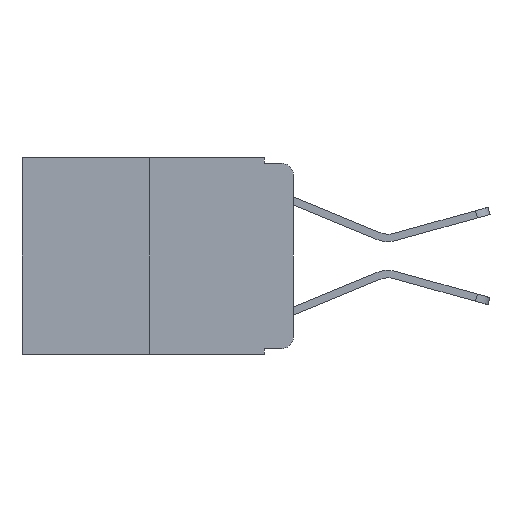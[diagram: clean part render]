
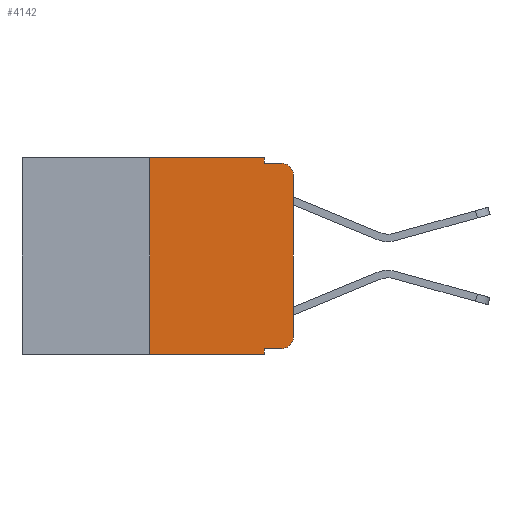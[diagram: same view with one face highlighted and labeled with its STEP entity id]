
A CAD part, left-side view. The second image highlights one B-rep face of the part: STEP entity #4142.
In plain terms, the highlighted planar face has unit normal (-1, 0, 0).
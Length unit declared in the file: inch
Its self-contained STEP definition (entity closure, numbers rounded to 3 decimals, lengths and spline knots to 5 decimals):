
#37 = DIRECTION ( 'NONE',  ( 0., -1., 0. ) ) ;
#138 = VECTOR ( 'NONE', #4565, 39.37008 ) ;
#332 = VERTEX_POINT ( 'NONE', #5326 ) ;
#410 = ORIENTED_EDGE ( 'NONE', *, *, #5003, .F. ) ;
#498 = VECTOR ( 'NONE', #1912, 39.37008 ) ;
#729 = EDGE_CURVE ( 'NONE', #332, #1767, #4614, .T. ) ;
#744 = LINE ( 'NONE', #3765, #852 ) ;
#795 = DIRECTION ( 'NONE',  ( 0., -1., 0. ) ) ;
#852 = VECTOR ( 'NONE', #9876, 39.37008 ) ;
#987 = EDGE_CURVE ( 'NONE', #9604, #3846, #1211, .T. ) ;
#1060 = CARTESIAN_POINT ( 'NONE',  ( 0., 0., 0. ) ) ;
#1211 = LINE ( 'NONE', #1060, #498 ) ;
#1225 = DIRECTION ( 'NONE',  ( 0., 0., -1. ) ) ;
#1314 = CARTESIAN_POINT ( 'NONE',  ( 0., 0.02, -0.03 ) ) ;
#1370 = PLANE ( 'NONE',  #2198 ) ;
#1767 = VERTEX_POINT ( 'NONE', #5515 ) ;
#1862 = ORIENTED_EDGE ( 'NONE', *, *, #2819, .F. ) ;
#1912 = DIRECTION ( 'NONE',  ( 0., 0., 1. ) ) ;
#2183 = EDGE_CURVE ( 'NONE', #1767, #5302, #744, .T. ) ;
#2198 = AXIS2_PLACEMENT_3D ( 'NONE', #9045, #6063, #7511 ) ;
#2219 = VECTOR ( 'NONE', #37, 39.37008 ) ;
#2294 = CARTESIAN_POINT ( 'NONE',  ( 0., 0.051, -0.01 ) ) ;
#2358 = LINE ( 'NONE', #4628, #5324 ) ;
#2541 = LINE ( 'NONE', #4808, #7480 ) ;
#2587 = DIRECTION ( 'NONE',  ( 0., 0., -1. ) ) ;
#2742 = ORIENTED_EDGE ( 'NONE', *, *, #3540, .T. ) ;
#2819 = EDGE_CURVE ( 'NONE', #7942, #332, #5285, .T. ) ;
#2828 = DIRECTION ( 'NONE',  ( 0., 0., 1. ) ) ;
#2835 = CIRCLE ( 'NONE', #9376, 0.02 ) ;
#2841 = DIRECTION ( 'NONE',  ( 0., 0., -1. ) ) ;
#3342 = EDGE_CURVE ( 'NONE', #9319, #7712, #2541, .T. ) ;
#3540 = EDGE_CURVE ( 'NONE', #7243, #9604, #2835, .T. ) ;
#3765 = CARTESIAN_POINT ( 'NONE',  ( 0., 0.051, 0. ) ) ;
#3846 = VERTEX_POINT ( 'NONE', #4092 ) ;
#3925 = CARTESIAN_POINT ( 'NONE',  ( 0., 0.051, -0.333 ) ) ;
#4092 = CARTESIAN_POINT ( 'NONE',  ( 0., 0., -0.03 ) ) ;
#4142 = ADVANCED_FACE ( 'NONE', ( #7606 ), #1370, .F. ) ;
#4565 = DIRECTION ( 'NONE',  ( 0., -1., 0. ) ) ;
#4577 = CARTESIAN_POINT ( 'NONE',  ( 0., 0., -0.313 ) ) ;
#4614 = LINE ( 'NONE', #5931, #7427 ) ;
#4628 = CARTESIAN_POINT ( 'NONE',  ( 0., 0.051, -0.333 ) ) ;
#4680 = ORIENTED_EDGE ( 'NONE', *, *, #2183, .F. ) ;
#4808 = CARTESIAN_POINT ( 'NONE',  ( 0., 0.051, 0. ) ) ;
#5003 = EDGE_CURVE ( 'NONE', #5302, #6569, #8308, .T. ) ;
#5243 = CARTESIAN_POINT ( 'NONE',  ( 0., 0.25, 0. ) ) ;
#5263 = EDGE_CURVE ( 'NONE', #3846, #6569, #6538, .T. ) ;
#5285 = LINE ( 'NONE', #5243, #8584 ) ;
#5302 = VERTEX_POINT ( 'NONE', #8946 ) ;
#5324 = VECTOR ( 'NONE', #795, 39.37008 ) ;
#5326 = CARTESIAN_POINT ( 'NONE',  ( 0., 0.25, 0. ) ) ;
#5469 = EDGE_CURVE ( 'NONE', #7942, #7712, #7744, .T. ) ;
#5515 = CARTESIAN_POINT ( 'NONE',  ( 0., 0.051, 0. ) ) ;
#5931 = CARTESIAN_POINT ( 'NONE',  ( 0., 0.473, 0. ) ) ;
#6063 = DIRECTION ( 'NONE',  ( 1., 0., 0. ) ) ;
#6495 = EDGE_LOOP ( 'NONE', ( #9462, #9490, #410, #4680, #9770, #1862, #7767, #6868, #8357, #2742 ) ) ;
#6538 = CIRCLE ( 'NONE', #7803, 0.02 ) ;
#6569 = VERTEX_POINT ( 'NONE', #9307 ) ;
#6708 = DIRECTION ( 'NONE',  ( -1., 0., 0. ) ) ;
#6868 = ORIENTED_EDGE ( 'NONE', *, *, #3342, .F. ) ;
#7243 = VERTEX_POINT ( 'NONE', #8706 ) ;
#7427 = VECTOR ( 'NONE', #7663, 39.37008 ) ;
#7474 = DIRECTION ( 'NONE',  ( -1., 0., 0. ) ) ;
#7480 = VECTOR ( 'NONE', #2587, 39.37008 ) ;
#7511 = DIRECTION ( 'NONE',  ( 0., 0., -1. ) ) ;
#7590 = CARTESIAN_POINT ( 'NONE',  ( 0., 0.25, -0.343 ) ) ;
#7606 = FACE_OUTER_BOUND ( 'NONE', #6495, .T. ) ;
#7663 = DIRECTION ( 'NONE',  ( 0., -1., 0. ) ) ;
#7712 = VERTEX_POINT ( 'NONE', #8525 ) ;
#7744 = LINE ( 'NONE', #9802, #2219 ) ;
#7767 = ORIENTED_EDGE ( 'NONE', *, *, #5469, .T. ) ;
#7803 = AXIS2_PLACEMENT_3D ( 'NONE', #1314, #6708, #2841 ) ;
#7942 = VERTEX_POINT ( 'NONE', #7590 ) ;
#8110 = CARTESIAN_POINT ( 'NONE',  ( 0., 0.02, -0.313 ) ) ;
#8308 = LINE ( 'NONE', #2294, #138 ) ;
#8357 = ORIENTED_EDGE ( 'NONE', *, *, #9747, .T. ) ;
#8525 = CARTESIAN_POINT ( 'NONE',  ( 0., 0.051, -0.343 ) ) ;
#8584 = VECTOR ( 'NONE', #2828, 39.37008 ) ;
#8706 = CARTESIAN_POINT ( 'NONE',  ( 0., 0.02, -0.333 ) ) ;
#8946 = CARTESIAN_POINT ( 'NONE',  ( 0., 0.051, -0.01 ) ) ;
#9045 = CARTESIAN_POINT ( 'NONE',  ( 0., 0.473, 0. ) ) ;
#9307 = CARTESIAN_POINT ( 'NONE',  ( 0., 0.02, -0.01 ) ) ;
#9319 = VERTEX_POINT ( 'NONE', #3925 ) ;
#9376 = AXIS2_PLACEMENT_3D ( 'NONE', #8110, #7474, #1225 ) ;
#9462 = ORIENTED_EDGE ( 'NONE', *, *, #987, .T. ) ;
#9490 = ORIENTED_EDGE ( 'NONE', *, *, #5263, .T. ) ;
#9604 = VERTEX_POINT ( 'NONE', #4577 ) ;
#9747 = EDGE_CURVE ( 'NONE', #9319, #7243, #2358, .T. ) ;
#9770 = ORIENTED_EDGE ( 'NONE', *, *, #729, .F. ) ;
#9802 = CARTESIAN_POINT ( 'NONE',  ( 0., 0.473, -0.343 ) ) ;
#9876 = DIRECTION ( 'NONE',  ( 0., 0., -1. ) ) ;
